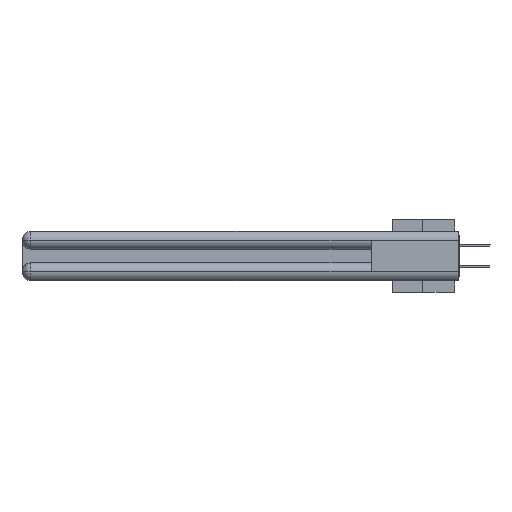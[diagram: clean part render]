
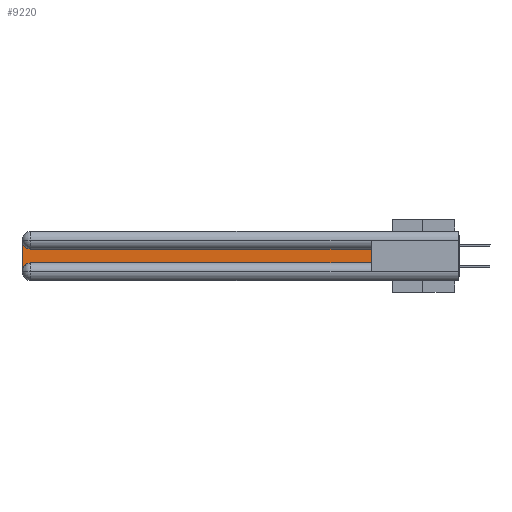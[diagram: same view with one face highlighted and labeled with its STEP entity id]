
A CAD part, left-side view. The second image highlights one B-rep face of the part: STEP entity #9220.
In plain terms, the highlighted planar face has unit normal (-1, 0, 0).
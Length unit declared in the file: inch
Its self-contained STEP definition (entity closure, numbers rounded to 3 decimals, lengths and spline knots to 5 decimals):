
#406 = EDGE_CURVE ( 'NONE', #5171, #11538, #29455, .T. ) ;
#770 = CARTESIAN_POINT ( 'NONE',  ( 0.075, 3., -0.1225 ) ) ;
#953 = DIRECTION ( 'NONE',  ( 0., -1., 0. ) ) ;
#1175 = DIRECTION ( 'NONE',  ( 0., 0., -1. ) ) ;
#1337 = AXIS2_PLACEMENT_3D ( 'NONE', #38581, #25348, #18666 ) ;
#4126 = LINE ( 'NONE', #26509, #21504 ) ;
#5171 = VERTEX_POINT ( 'NONE', #25314 ) ;
#5578 = AXIS2_PLACEMENT_3D ( 'NONE', #770, #33040, #7071 ) ;
#6324 = ORIENTED_EDGE ( 'NONE', *, *, #42135, .T. ) ;
#7071 = DIRECTION ( 'NONE',  ( 0., 0., -1. ) ) ;
#8091 = CARTESIAN_POINT ( 'NONE',  ( 0.075, 0.6, -0.1225 ) ) ;
#8612 = ORIENTED_EDGE ( 'NONE', *, *, #24829, .T. ) ;
#9220 = ADVANCED_FACE ( 'NONE', ( #25720 ), #26611, .F. ) ;
#10288 = CIRCLE ( 'NONE', #1337, 0.06 ) ;
#11208 = CARTESIAN_POINT ( 'NONE',  ( 0.075, 3., -0.2175 ) ) ;
#11538 = VERTEX_POINT ( 'NONE', #8091 ) ;
#12143 = VECTOR ( 'NONE', #22008, 39.37008 ) ;
#15290 = CARTESIAN_POINT ( 'NONE',  ( 0.075, 2.94, -0.2175 ) ) ;
#15709 = EDGE_CURVE ( 'NONE', #39754, #32522, #35080, .T. ) ;
#18666 = DIRECTION ( 'NONE',  ( 0., 0., -1. ) ) ;
#20732 = DIRECTION ( 'NONE',  ( 1., 0., 0. ) ) ;
#21437 = VERTEX_POINT ( 'NONE', #31509 ) ;
#21504 = VECTOR ( 'NONE', #953, 39.37008 ) ;
#22008 = DIRECTION ( 'NONE',  ( 0., 0., 1. ) ) ;
#23194 = CARTESIAN_POINT ( 'NONE',  ( 0.075, 0.6, -0.1225 ) ) ;
#23227 = LINE ( 'NONE', #23194, #34972 ) ;
#23737 = CARTESIAN_POINT ( 'NONE',  ( 0.075, 2.94, -0.2775 ) ) ;
#24498 = VERTEX_POINT ( 'NONE', #15290 ) ;
#24552 = CARTESIAN_POINT ( 'NONE',  ( 0.075, 3., -0.0625 ) ) ;
#24829 = EDGE_CURVE ( 'NONE', #24498, #5171, #4126, .T. ) ;
#25076 = ORIENTED_EDGE ( 'NONE', *, *, #39080, .T. ) ;
#25314 = CARTESIAN_POINT ( 'NONE',  ( 0.075, 0.6, -0.2175 ) ) ;
#25348 = DIRECTION ( 'NONE',  ( 1., 0., 0. ) ) ;
#25720 = FACE_OUTER_BOUND ( 'NONE', #36132, .T. ) ;
#26332 = DIRECTION ( 'NONE',  ( 0., 1., 0. ) ) ;
#26509 = CARTESIAN_POINT ( 'NONE',  ( 0.075, 0.6, -0.2175 ) ) ;
#26611 = PLANE ( 'NONE',  #5578 ) ;
#26891 = VECTOR ( 'NONE', #1175, 39.37008 ) ;
#27128 = AXIS2_PLACEMENT_3D ( 'NONE', #23737, #20732, #27281 ) ;
#27281 = DIRECTION ( 'NONE',  ( 0., 0., -1. ) ) ;
#28735 = ORIENTED_EDGE ( 'NONE', *, *, #35813, .T. ) ;
#29455 = LINE ( 'NONE', #38089, #12143 ) ;
#29945 = CARTESIAN_POINT ( 'NONE',  ( 0.075, 3., -0.2775 ) ) ;
#31509 = CARTESIAN_POINT ( 'NONE',  ( 0.075, 2.94, -0.1225 ) ) ;
#31610 = ORIENTED_EDGE ( 'NONE', *, *, #406, .T. ) ;
#32522 = VERTEX_POINT ( 'NONE', #29945 ) ;
#33040 = DIRECTION ( 'NONE',  ( 1., 0., 0. ) ) ;
#34972 = VECTOR ( 'NONE', #26332, 39.37008 ) ;
#35080 = LINE ( 'NONE', #11208, #26891 ) ;
#35813 = EDGE_CURVE ( 'NONE', #21437, #39754, #10288, .T. ) ;
#36132 = EDGE_LOOP ( 'NONE', ( #6324, #28735, #36792, #25076, #8612, #31610 ) ) ;
#36161 = CIRCLE ( 'NONE', #27128, 0.06 ) ;
#36792 = ORIENTED_EDGE ( 'NONE', *, *, #15709, .T. ) ;
#38089 = CARTESIAN_POINT ( 'NONE',  ( 0.075, 0.6, -0.2175 ) ) ;
#38581 = CARTESIAN_POINT ( 'NONE',  ( 0.075, 2.94, -0.0625 ) ) ;
#39080 = EDGE_CURVE ( 'NONE', #32522, #24498, #36161, .T. ) ;
#39754 = VERTEX_POINT ( 'NONE', #24552 ) ;
#42135 = EDGE_CURVE ( 'NONE', #11538, #21437, #23227, .T. ) ;
